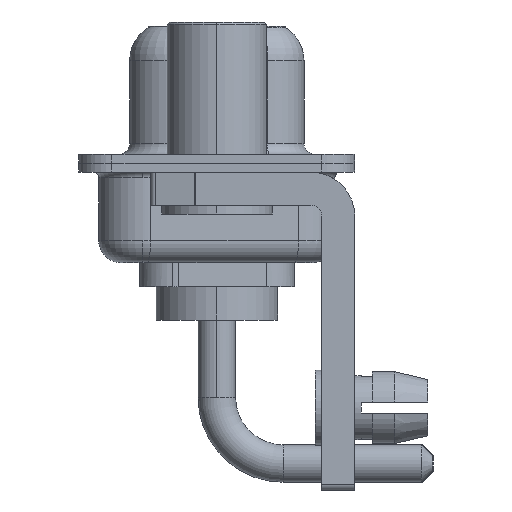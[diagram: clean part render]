
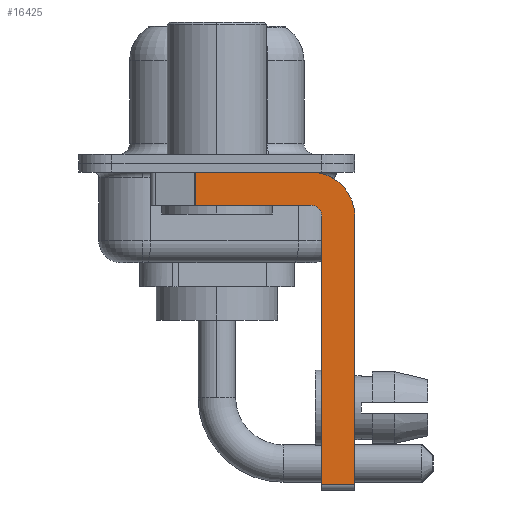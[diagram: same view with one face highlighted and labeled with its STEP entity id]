
A CAD part, left-side view. The second image highlights one B-rep face of the part: STEP entity #16425.
In plain terms, the highlighted planar face has unit normal (-1, 0, 0).
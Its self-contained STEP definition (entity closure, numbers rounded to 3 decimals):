
#104 = DIRECTION ( 'NONE',  ( 0., 0., -1. ) ) ;
#177 = CIRCLE ( 'NONE', #12774, 2. ) ;
#269 = DIRECTION ( 'NONE',  ( -1., 0., 0. ) ) ;
#286 = DIRECTION ( 'NONE',  ( 0., 0., 1. ) ) ;
#954 = VERTEX_POINT ( 'NONE', #11521 ) ;
#1180 = EDGE_LOOP ( 'NONE', ( #12675, #2245, #7103, #12791, #6092, #13928, #1195, #3635 ) ) ;
#1195 = ORIENTED_EDGE ( 'NONE', *, *, #4444, .F. ) ;
#1446 = CARTESIAN_POINT ( 'NONE',  ( -2.9, -6.25, -2.4 ) ) ;
#1523 = LINE ( 'NONE', #6959, #8495 ) ;
#1564 = CARTESIAN_POINT ( 'NONE',  ( -2.9, -6.25, -14.55 ) ) ;
#1774 = CARTESIAN_POINT ( 'NONE',  ( -2.9, -4.75, -14.8 ) ) ;
#1833 = VERTEX_POINT ( 'NONE', #1564 ) ;
#1979 = CARTESIAN_POINT ( 'NONE',  ( -2.9, 3., -0.4 ) ) ;
#2163 = LINE ( 'NONE', #11512, #10504 ) ;
#2165 = DIRECTION ( 'NONE',  ( 0., -1., 0. ) ) ;
#2245 = ORIENTED_EDGE ( 'NONE', *, *, #13758, .T. ) ;
#2637 = CARTESIAN_POINT ( 'NONE',  ( -2.9, 0.978, -1.9 ) ) ;
#2651 = VECTOR ( 'NONE', #2165, 1000. ) ;
#2820 = CARTESIAN_POINT ( 'NONE',  ( -2.9, -4.25, -1.9 ) ) ;
#3028 = LINE ( 'NONE', #1774, #9346 ) ;
#3216 = VERTEX_POINT ( 'NONE', #2820 ) ;
#3635 = ORIENTED_EDGE ( 'NONE', *, *, #10120, .F. ) ;
#4300 = DIRECTION ( 'NONE',  ( 0., 1., 0. ) ) ;
#4444 = EDGE_CURVE ( 'NONE', #16204, #1833, #1523, .T. ) ;
#4576 = CARTESIAN_POINT ( 'NONE',  ( -2.9, -4.25, -0.4 ) ) ;
#4912 = AXIS2_PLACEMENT_3D ( 'NONE', #12267, #269, #14737 ) ;
#4981 = CARTESIAN_POINT ( 'NONE',  ( -2.9, -4.25, -2.4 ) ) ;
#5452 = VECTOR ( 'NONE', #11323, 1000. ) ;
#5585 = DIRECTION ( 'NONE',  ( 0., 0., -1. ) ) ;
#6092 = ORIENTED_EDGE ( 'NONE', *, *, #13649, .F. ) ;
#6136 = EDGE_CURVE ( 'NONE', #17309, #3216, #9952, .T. ) ;
#6692 = EDGE_CURVE ( 'NONE', #954, #15561, #14140, .T. ) ;
#6959 = CARTESIAN_POINT ( 'NONE',  ( -2.9, -6.25, -2.4 ) ) ;
#7036 = FACE_OUTER_BOUND ( 'NONE', #1180, .T. ) ;
#7103 = ORIENTED_EDGE ( 'NONE', *, *, #7961, .F. ) ;
#7295 = CARTESIAN_POINT ( 'NONE',  ( -2.9, -4.25, -2.4 ) ) ;
#7655 = DIRECTION ( 'NONE',  ( 0., -1., 0. ) ) ;
#7961 = EDGE_CURVE ( 'NONE', #3216, #8238, #17344, .T. ) ;
#7986 = VECTOR ( 'NONE', #4300, 1000. ) ;
#8238 = VERTEX_POINT ( 'NONE', #2637 ) ;
#8495 = VECTOR ( 'NONE', #104, 1000. ) ;
#8624 = DIRECTION ( 'NONE',  ( 1., 0., 0. ) ) ;
#8915 = DIRECTION ( 'NONE',  ( 0., 0., -1. ) ) ;
#9042 = CARTESIAN_POINT ( 'NONE',  ( -2.9, -4.75, -14.55 ) ) ;
#9346 = VECTOR ( 'NONE', #286, 1000. ) ;
#9721 = CARTESIAN_POINT ( 'NONE',  ( -2.9, -4.75, -2.4 ) ) ;
#9952 = CIRCLE ( 'NONE', #4912, 0.5 ) ;
#10120 = EDGE_CURVE ( 'NONE', #15561, #16204, #177, .T. ) ;
#10504 = VECTOR ( 'NONE', #7655, 1000. ) ;
#11085 = AXIS2_PLACEMENT_3D ( 'NONE', #7295, #8624, #5585 ) ;
#11323 = DIRECTION ( 'NONE',  ( 0., 0., -1. ) ) ;
#11493 = LINE ( 'NONE', #15272, #5452 ) ;
#11512 = CARTESIAN_POINT ( 'NONE',  ( -2.9, -4.25, -14.55 ) ) ;
#11520 = DIRECTION ( 'NONE',  ( 1., 0., 0. ) ) ;
#11521 = CARTESIAN_POINT ( 'NONE',  ( -2.9, 0.978, -0.4 ) ) ;
#12267 = CARTESIAN_POINT ( 'NONE',  ( -2.9, -4.25, -2.4 ) ) ;
#12675 = ORIENTED_EDGE ( 'NONE', *, *, #6692, .F. ) ;
#12774 = AXIS2_PLACEMENT_3D ( 'NONE', #4981, #11520, #8915 ) ;
#12791 = ORIENTED_EDGE ( 'NONE', *, *, #6136, .F. ) ;
#13614 = PLANE ( 'NONE',  #11085 ) ;
#13649 = EDGE_CURVE ( 'NONE', #13906, #17309, #3028, .T. ) ;
#13758 = EDGE_CURVE ( 'NONE', #954, #8238, #11493, .T. ) ;
#13906 = VERTEX_POINT ( 'NONE', #9042 ) ;
#13928 = ORIENTED_EDGE ( 'NONE', *, *, #14688, .T. ) ;
#14140 = LINE ( 'NONE', #1979, #2651 ) ;
#14688 = EDGE_CURVE ( 'NONE', #13906, #1833, #2163, .T. ) ;
#14737 = DIRECTION ( 'NONE',  ( 0., 0., 1. ) ) ;
#15272 = CARTESIAN_POINT ( 'NONE',  ( -2.9, 0.978, -1.9 ) ) ;
#15561 = VERTEX_POINT ( 'NONE', #4576 ) ;
#16114 = CARTESIAN_POINT ( 'NONE',  ( -2.9, -4.25, -1.9 ) ) ;
#16204 = VERTEX_POINT ( 'NONE', #1446 ) ;
#16425 = ADVANCED_FACE ( 'NONE', ( #7036 ), #13614, .F. ) ;
#17309 = VERTEX_POINT ( 'NONE', #9721 ) ;
#17344 = LINE ( 'NONE', #16114, #7986 ) ;
